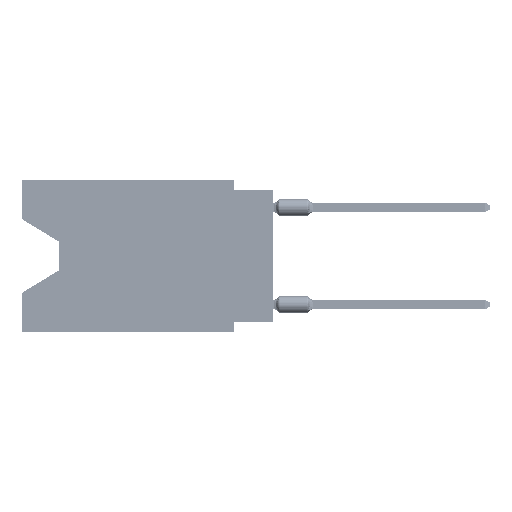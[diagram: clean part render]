
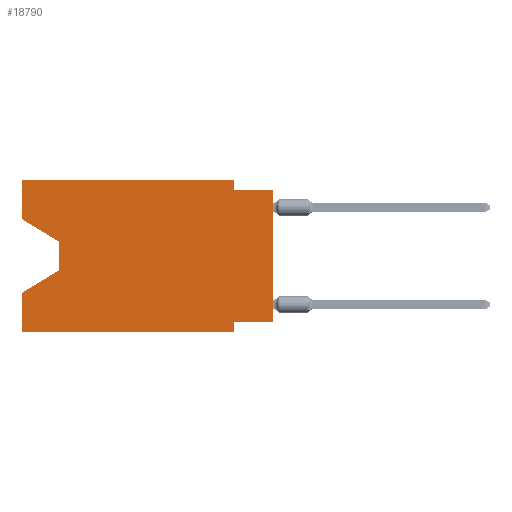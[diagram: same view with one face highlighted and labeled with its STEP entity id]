
A CAD part, left-side view. The second image highlights one B-rep face of the part: STEP entity #18790.
In plain terms, the highlighted planar face has unit normal (-1, 0, 0).
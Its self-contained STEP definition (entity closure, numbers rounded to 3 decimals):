
#669 = VECTOR ( 'NONE', #13393, 1000. ) ;
#903 = VERTEX_POINT ( 'NONE', #1033 ) ;
#1033 = CARTESIAN_POINT ( 'NONE',  ( 0., 13.97, -5.893 ) ) ;
#2021 = LINE ( 'NONE', #36290, #53838 ) ;
#2129 = LINE ( 'NONE', #25986, #55548 ) ;
#2346 = LINE ( 'NONE', #67355, #37454 ) ;
#2545 = LINE ( 'NONE', #72953, #51316 ) ;
#5008 = EDGE_CURVE ( 'NONE', #5346, #43169, #2545, .T. ) ;
#5346 = VERTEX_POINT ( 'NONE', #50524 ) ;
#6565 = EDGE_LOOP ( 'NONE', ( #39487, #56736, #31045, #28745, #75426, #26533, #7378, #12547, #71836, #52584, #26296, #16355 ) ) ;
#7134 = CARTESIAN_POINT ( 'NONE',  ( 0., 13.97, -4.013 ) ) ;
#7378 = ORIENTED_EDGE ( 'NONE', *, *, #33807, .F. ) ;
#7725 = DIRECTION ( 'NONE',  ( 0., 0., 1. ) ) ;
#9639 = VERTEX_POINT ( 'NONE', #37111 ) ;
#9894 = CARTESIAN_POINT ( 'NONE',  ( 0., 16.383, 0. ) ) ;
#11517 = DIRECTION ( 'NONE',  ( 0., 1., 0. ) ) ;
#11886 = CARTESIAN_POINT ( 'NONE',  ( 0., 0., -9.271 ) ) ;
#12547 = ORIENTED_EDGE ( 'NONE', *, *, #30506, .T. ) ;
#13393 = DIRECTION ( 'NONE',  ( 0., 0., -1. ) ) ;
#16355 = ORIENTED_EDGE ( 'NONE', *, *, #48072, .F. ) ;
#16788 = DIRECTION ( 'NONE',  ( 0., 0., 1. ) ) ;
#17072 = AXIS2_PLACEMENT_3D ( 'NONE', #74644, #28465, #21568 ) ;
#18216 = VERTEX_POINT ( 'NONE', #32452 ) ;
#18790 = ADVANCED_FACE ( 'NONE', ( #45419 ), #26961, .F. ) ;
#19154 = LINE ( 'NONE', #48008, #669 ) ;
#20255 = DIRECTION ( 'NONE',  ( 0., -1., 0. ) ) ;
#21187 = DIRECTION ( 'NONE',  ( 0., 0., 1. ) ) ;
#21568 = DIRECTION ( 'NONE',  ( 0., 0., -1. ) ) ;
#22699 = VERTEX_POINT ( 'NONE', #38324 ) ;
#22891 = EDGE_CURVE ( 'NONE', #42208, #61596, #2021, .T. ) ;
#24826 = CARTESIAN_POINT ( 'NONE',  ( 0., 13.97, -4.013 ) ) ;
#25986 = CARTESIAN_POINT ( 'NONE',  ( 0., 13.97, -5.893 ) ) ;
#26296 = ORIENTED_EDGE ( 'NONE', *, *, #48804, .F. ) ;
#26533 = ORIENTED_EDGE ( 'NONE', *, *, #41280, .F. ) ;
#26961 = PLANE ( 'NONE',  #17072 ) ;
#28233 = VECTOR ( 'NONE', #43209, 1000. ) ;
#28465 = DIRECTION ( 'NONE',  ( 1., 0., 0. ) ) ;
#28745 = ORIENTED_EDGE ( 'NONE', *, *, #59919, .F. ) ;
#30506 = EDGE_CURVE ( 'NONE', #18216, #66805, #30823, .T. ) ;
#30823 = LINE ( 'NONE', #60819, #38869 ) ;
#31045 = ORIENTED_EDGE ( 'NONE', *, *, #34402, .T. ) ;
#32452 = CARTESIAN_POINT ( 'NONE',  ( 0., 0., -9.271 ) ) ;
#32670 = DIRECTION ( 'NONE',  ( 0., -1., 0. ) ) ;
#33807 = EDGE_CURVE ( 'NONE', #18216, #40731, #59562, .T. ) ;
#33999 = CARTESIAN_POINT ( 'NONE',  ( 0., 2.54, -9.906 ) ) ;
#34402 = EDGE_CURVE ( 'NONE', #903, #9639, #2129, .T. ) ;
#36290 = CARTESIAN_POINT ( 'NONE',  ( 0., 16.383, -2.546 ) ) ;
#37111 = CARTESIAN_POINT ( 'NONE',  ( 0., 16.383, -7.36 ) ) ;
#37454 = VECTOR ( 'NONE', #21187, 1000. ) ;
#38324 = CARTESIAN_POINT ( 'NONE',  ( 0., 2.54, 0. ) ) ;
#38869 = VECTOR ( 'NONE', #7725, 1000. ) ;
#39204 = VERTEX_POINT ( 'NONE', #42042 ) ;
#39487 = ORIENTED_EDGE ( 'NONE', *, *, #22891, .T. ) ;
#40731 = VERTEX_POINT ( 'NONE', #46218 ) ;
#40869 = VERTEX_POINT ( 'NONE', #49237 ) ;
#41280 = EDGE_CURVE ( 'NONE', #40731, #43169, #19154, .T. ) ;
#41633 = EDGE_CURVE ( 'NONE', #61596, #903, #65225, .T. ) ;
#42042 = CARTESIAN_POINT ( 'NONE',  ( 0., 2.54, -0.635 ) ) ;
#42208 = VERTEX_POINT ( 'NONE', #72430 ) ;
#42554 = DIRECTION ( 'NONE',  ( 0., 0.855, -0.519 ) ) ;
#43169 = VERTEX_POINT ( 'NONE', #33999 ) ;
#43198 = DIRECTION ( 'NONE',  ( 0., -0.855, -0.519 ) ) ;
#43209 = DIRECTION ( 'NONE',  ( 0., -1., 0. ) ) ;
#44486 = VECTOR ( 'NONE', #32670, 1000. ) ;
#45419 = FACE_OUTER_BOUND ( 'NONE', #6565, .T. ) ;
#46218 = CARTESIAN_POINT ( 'NONE',  ( 0., 2.54, -9.271 ) ) ;
#46265 = CARTESIAN_POINT ( 'NONE',  ( 0., 0., -0.635 ) ) ;
#48008 = CARTESIAN_POINT ( 'NONE',  ( 0., 2.54, -9.906 ) ) ;
#48072 = EDGE_CURVE ( 'NONE', #42208, #40869, #57571, .T. ) ;
#48804 = EDGE_CURVE ( 'NONE', #40869, #22699, #72816, .T. ) ;
#49237 = CARTESIAN_POINT ( 'NONE',  ( 0., 16.383, 0. ) ) ;
#50524 = CARTESIAN_POINT ( 'NONE',  ( 0., 16.383, -9.906 ) ) ;
#51111 = LINE ( 'NONE', #61895, #44486 ) ;
#51316 = VECTOR ( 'NONE', #20255, 1000. ) ;
#52584 = ORIENTED_EDGE ( 'NONE', *, *, #71910, .F. ) ;
#53408 = EDGE_CURVE ( 'NONE', #39204, #66805, #51111, .T. ) ;
#53838 = VECTOR ( 'NONE', #43198, 1000. ) ;
#55548 = VECTOR ( 'NONE', #42554, 1000. ) ;
#56736 = ORIENTED_EDGE ( 'NONE', *, *, #41633, .T. ) ;
#57571 = LINE ( 'NONE', #9894, #60089 ) ;
#59347 = VECTOR ( 'NONE', #11517, 1000. ) ;
#59562 = LINE ( 'NONE', #11886, #59347 ) ;
#59919 = EDGE_CURVE ( 'NONE', #5346, #9639, #2346, .T. ) ;
#60089 = VECTOR ( 'NONE', #16788, 1000. ) ;
#60819 = CARTESIAN_POINT ( 'NONE',  ( 0., 0., 0. ) ) ;
#61596 = VERTEX_POINT ( 'NONE', #7134 ) ;
#61895 = CARTESIAN_POINT ( 'NONE',  ( 0., 0., -0.635 ) ) ;
#64479 = DIRECTION ( 'NONE',  ( 0., 0., -1. ) ) ;
#64649 = VECTOR ( 'NONE', #64479, 1000. ) ;
#65225 = LINE ( 'NONE', #24826, #64649 ) ;
#65411 = DIRECTION ( 'NONE',  ( 0., 0., -1. ) ) ;
#66542 = LINE ( 'NONE', #71554, #71562 ) ;
#66805 = VERTEX_POINT ( 'NONE', #46265 ) ;
#67035 = CARTESIAN_POINT ( 'NONE',  ( 0., 16.383, 0. ) ) ;
#67355 = CARTESIAN_POINT ( 'NONE',  ( 0., 16.383, 0. ) ) ;
#71554 = CARTESIAN_POINT ( 'NONE',  ( 0., 2.54, 0. ) ) ;
#71562 = VECTOR ( 'NONE', #65411, 1000. ) ;
#71836 = ORIENTED_EDGE ( 'NONE', *, *, #53408, .F. ) ;
#71910 = EDGE_CURVE ( 'NONE', #22699, #39204, #66542, .T. ) ;
#72430 = CARTESIAN_POINT ( 'NONE',  ( 0., 16.383, -2.546 ) ) ;
#72816 = LINE ( 'NONE', #67035, #28233 ) ;
#72953 = CARTESIAN_POINT ( 'NONE',  ( 0., 16.383, -9.906 ) ) ;
#74644 = CARTESIAN_POINT ( 'NONE',  ( 0., 16.383, 0. ) ) ;
#75426 = ORIENTED_EDGE ( 'NONE', *, *, #5008, .T. ) ;
